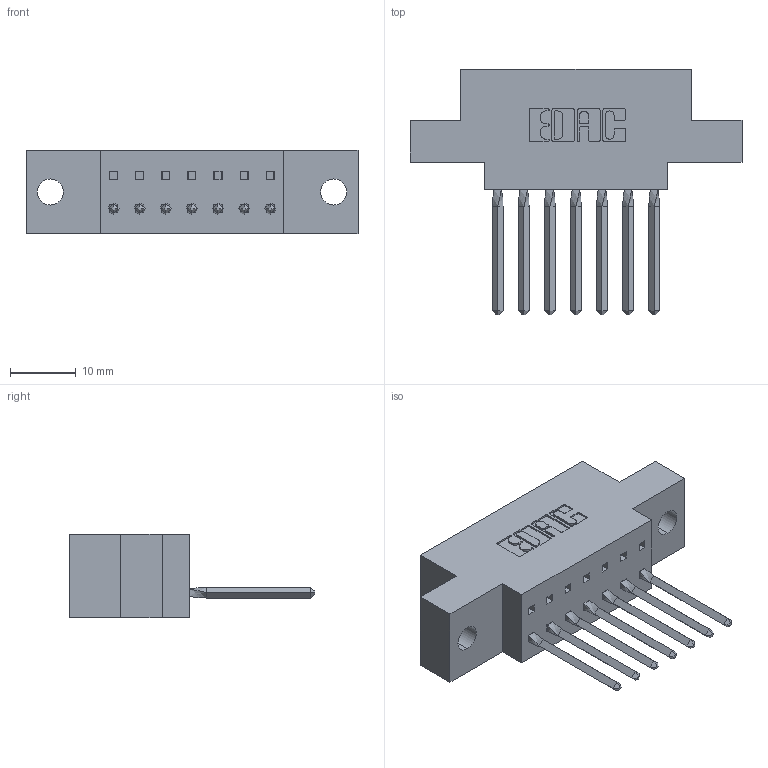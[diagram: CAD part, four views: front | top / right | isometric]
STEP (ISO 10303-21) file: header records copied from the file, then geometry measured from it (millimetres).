
FILE_DESCRIPTION (( 'STEP AP203' ), '1' );
FILE_NAME ('317-007-541-604.STEP', '2020-02-27T12:57:51', ( '' ), ( '' ), 'SwSTEP 2.0', 'SolidWorks 2016', '' );
FILE_SCHEMA (( 'CONFIG_CONTROL_DESIGN' ));
Length unit declared in the file: inch
Products named in the file (3): 317-290-002_541; 317 Part_.156 Dia - TH; 317-007-541-604
Assembly tree (8 placements, depth 2):
  317-007-541-604
    317 Part_.156 Dia - TH
    317-290-002_541  x7
Bounding box: 50.44 x 37.34 x 12.7 mm (x, y, z)
Volume: 7016.3 mm3; surface area: 8565.7 mm2
Topology: 8 solids, 8 shells, 1166 faces, 3313 edges, 2156 vertices
Faces by surface type: plane 926, cylinder 212, bspline 28
Entity records: 16328 total; most frequent: CARTESIAN_POINT 3526, ORIENTED_EDGE 2786, DIRECTION 2263, EDGE_CURVE 1393, LINE 1029, VECTOR 1029, VERTEX_POINT 920, AXIS2_PLACEMENT_3D 617
